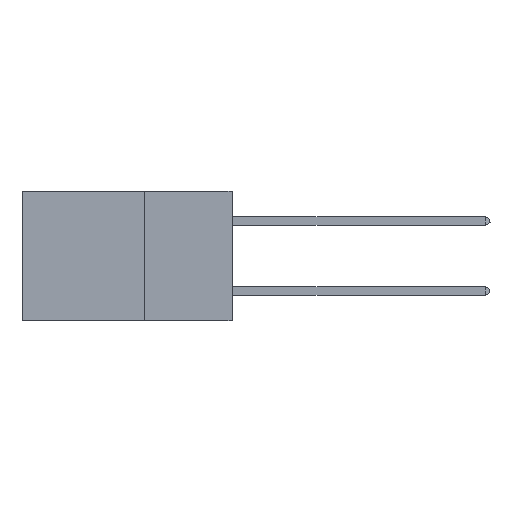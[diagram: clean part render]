
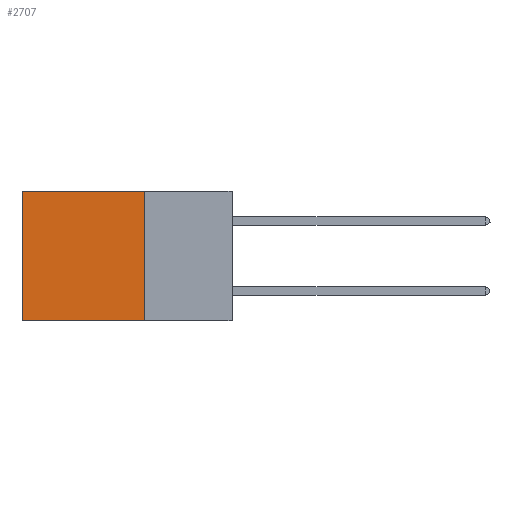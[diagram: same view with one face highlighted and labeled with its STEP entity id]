
A CAD part, left-side view. The second image highlights one B-rep face of the part: STEP entity #2707.
In plain terms, the highlighted planar face has unit normal (-1, 0, 0).
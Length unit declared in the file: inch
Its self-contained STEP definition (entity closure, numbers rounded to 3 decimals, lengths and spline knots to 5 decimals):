
#299 = EDGE_CURVE ( 'NONE', #2751, #8400, #14090, .T. ) ;
#1672 = CARTESIAN_POINT ( 'NONE',  ( 0.2875, 0.25, 0. ) ) ;
#2707 = ADVANCED_FACE ( 'NONE', ( #19404 ), #29205, .F. ) ;
#2751 = VERTEX_POINT ( 'NONE', #11479 ) ;
#3638 = DIRECTION ( 'NONE',  ( 0., 0., -1. ) ) ;
#3787 = VERTEX_POINT ( 'NONE', #9721 ) ;
#3838 = VECTOR ( 'NONE', #3638, 39.37008 ) ;
#4475 = DIRECTION ( 'NONE',  ( 0., 0., -1. ) ) ;
#4479 = ORIENTED_EDGE ( 'NONE', *, *, #22577, .T. ) ;
#5501 = CARTESIAN_POINT ( 'NONE',  ( 0.2875, 0.6, 0. ) ) ;
#5535 = VECTOR ( 'NONE', #16882, 39.37008 ) ;
#6869 = VECTOR ( 'NONE', #11059, 39.37008 ) ;
#6992 = CARTESIAN_POINT ( 'NONE',  ( 0.2875, 0.25, 0. ) ) ;
#7433 = ORIENTED_EDGE ( 'NONE', *, *, #15626, .F. ) ;
#8400 = VERTEX_POINT ( 'NONE', #19909 ) ;
#8777 = AXIS2_PLACEMENT_3D ( 'NONE', #11788, #19562, #4475 ) ;
#9103 = CARTESIAN_POINT ( 'NONE',  ( 0.2875, 0.25, 0. ) ) ;
#9664 = VERTEX_POINT ( 'NONE', #1672 ) ;
#9721 = CARTESIAN_POINT ( 'NONE',  ( 0.2875, 0.25, -0.37 ) ) ;
#11059 = DIRECTION ( 'NONE',  ( 0., 1., 0. ) ) ;
#11479 = CARTESIAN_POINT ( 'NONE',  ( 0.2875, 0.6, 0. ) ) ;
#11788 = CARTESIAN_POINT ( 'NONE',  ( 0.2875, 0.25, 0. ) ) ;
#12429 = LINE ( 'NONE', #32667, #23561 ) ;
#13851 = LINE ( 'NONE', #6992, #6869 ) ;
#14090 = LINE ( 'NONE', #5501, #3838 ) ;
#14904 = DIRECTION ( 'NONE',  ( 0., 1., 0. ) ) ;
#15626 = EDGE_CURVE ( 'NONE', #9664, #3787, #24358, .T. ) ;
#16685 = EDGE_LOOP ( 'NONE', ( #17320, #30691, #7433, #4479 ) ) ;
#16882 = DIRECTION ( 'NONE',  ( 0., 0., -1. ) ) ;
#17320 = ORIENTED_EDGE ( 'NONE', *, *, #299, .T. ) ;
#19404 = FACE_OUTER_BOUND ( 'NONE', #16685, .T. ) ;
#19562 = DIRECTION ( 'NONE',  ( 1., 0., 0. ) ) ;
#19909 = CARTESIAN_POINT ( 'NONE',  ( 0.2875, 0.6, -0.37 ) ) ;
#22577 = EDGE_CURVE ( 'NONE', #9664, #2751, #13851, .T. ) ;
#23561 = VECTOR ( 'NONE', #14904, 39.37008 ) ;
#24358 = LINE ( 'NONE', #9103, #5535 ) ;
#29205 = PLANE ( 'NONE',  #8777 ) ;
#30198 = EDGE_CURVE ( 'NONE', #3787, #8400, #12429, .T. ) ;
#30691 = ORIENTED_EDGE ( 'NONE', *, *, #30198, .F. ) ;
#32667 = CARTESIAN_POINT ( 'NONE',  ( 0.2875, 0.25, -0.37 ) ) ;
